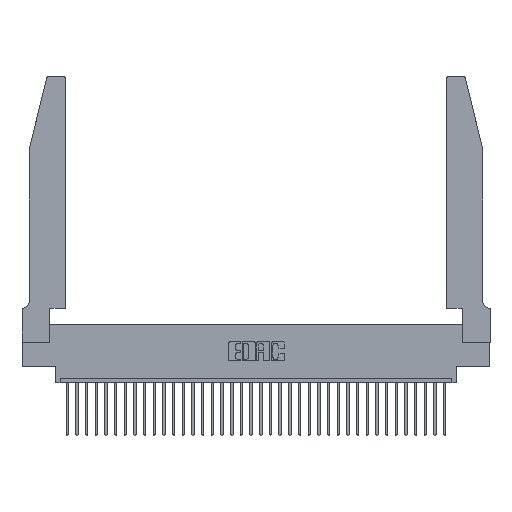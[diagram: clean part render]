
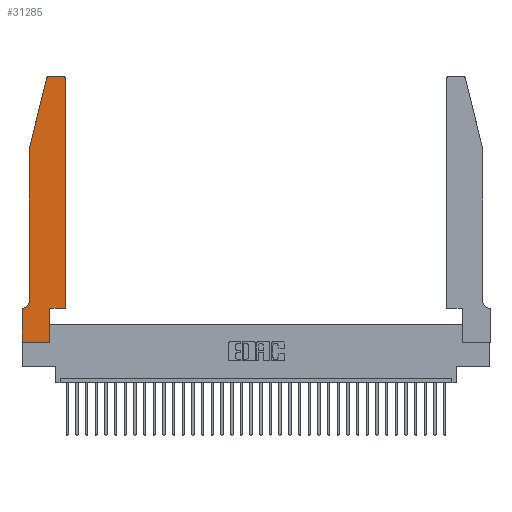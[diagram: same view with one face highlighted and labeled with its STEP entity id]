
A CAD part, top view. The second image highlights one B-rep face of the part: STEP entity #31285.
In plain terms, the highlighted planar face has unit normal (0, 0, 1).
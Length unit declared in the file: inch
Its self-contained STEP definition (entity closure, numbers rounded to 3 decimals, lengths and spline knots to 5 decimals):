
#477 = VECTOR ( 'NONE', #29769, 39.37008 ) ;
#1141 = ORIENTED_EDGE ( 'NONE', *, *, #14739, .T. ) ;
#1378 = EDGE_CURVE ( 'NONE', #14577, #11695, #32129, .T. ) ;
#1543 = EDGE_CURVE ( 'NONE', #13405, #30024, #4927, .T. ) ;
#3015 = DIRECTION ( 'NONE',  ( 0., -1., 0. ) ) ;
#3375 = ORIENTED_EDGE ( 'NONE', *, *, #1543, .T. ) ;
#3447 = CARTESIAN_POINT ( 'NONE',  ( 0.0755, 2., 0.37 ) ) ;
#3746 = EDGE_CURVE ( 'NONE', #33230, #19963, #22677, .T. ) ;
#3959 = EDGE_CURVE ( 'NONE', #5600, #13405, #12819, .T. ) ;
#4927 = LINE ( 'NONE', #29411, #30412 ) ;
#5176 = CARTESIAN_POINT ( 'NONE',  ( 0.2605, 2.75, 0.37 ) ) ;
#5201 = CARTESIAN_POINT ( 'NONE',  ( 0.4205, 2.72, 0.37 ) ) ;
#5505 = CARTESIAN_POINT ( 'NONE',  ( 0.4505, 0.35, 0.37 ) ) ;
#5600 = VERTEX_POINT ( 'NONE', #30991 ) ;
#5765 = FACE_OUTER_BOUND ( 'NONE', #14276, .T. ) ;
#5820 = CARTESIAN_POINT ( 'NONE',  ( 0.25487, 2.72718, 0.37 ) ) ;
#6359 = CARTESIAN_POINT ( 'NONE',  ( 0., 0., 0.37 ) ) ;
#6384 = DIRECTION ( 'NONE',  ( 0., 0., 1. ) ) ;
#6611 = VECTOR ( 'NONE', #15570, 39.37008 ) ;
#6626 = DIRECTION ( 'NONE',  ( 1., 0., 0. ) ) ;
#7242 = ORIENTED_EDGE ( 'NONE', *, *, #23865, .T. ) ;
#7427 = CARTESIAN_POINT ( 'NONE',  ( 0., 0., 0.37 ) ) ;
#8271 = CARTESIAN_POINT ( 'NONE',  ( 0.0755, 0.42, 0.37 ) ) ;
#8273 = LINE ( 'NONE', #5176, #6611 ) ;
#8290 = CARTESIAN_POINT ( 'NONE',  ( 0.0055, 0.35, 0.37 ) ) ;
#8699 = EDGE_CURVE ( 'NONE', #32568, #24597, #12041, .T. ) ;
#9006 = EDGE_CURVE ( 'NONE', #24597, #27833, #17996, .T. ) ;
#9577 = DIRECTION ( 'NONE',  ( 0., -1., 0. ) ) ;
#9740 = AXIS2_PLACEMENT_3D ( 'NONE', #5201, #16184, #10768 ) ;
#10243 = EDGE_CURVE ( 'NONE', #19963, #14577, #11085, .T. ) ;
#10768 = DIRECTION ( 'NONE',  ( 1., 0., 0. ) ) ;
#11085 = LINE ( 'NONE', #28602, #31528 ) ;
#11299 = AXIS2_PLACEMENT_3D ( 'NONE', #27992, #6384, #6626 ) ;
#11360 = CARTESIAN_POINT ( 'NONE',  ( 0., 0.35, 0.37 ) ) ;
#11546 = ORIENTED_EDGE ( 'NONE', *, *, #1378, .T. ) ;
#11695 = VERTEX_POINT ( 'NONE', #32673 ) ;
#12041 = CIRCLE ( 'NONE', #25523, 0.03 ) ;
#12495 = VECTOR ( 'NONE', #30322, 39.37008 ) ;
#12645 = CARTESIAN_POINT ( 'NONE',  ( 0.4205, 2.75, 0.37 ) ) ;
#12819 = LINE ( 'NONE', #29457, #25585 ) ;
#13137 = DIRECTION ( 'NONE',  ( 0., 1., 0. ) ) ;
#13267 = VECTOR ( 'NONE', #3015, 39.37008 ) ;
#13405 = VERTEX_POINT ( 'NONE', #5505 ) ;
#13444 = ORIENTED_EDGE ( 'NONE', *, *, #31544, .T. ) ;
#13888 = DIRECTION ( 'NONE',  ( -1., 0., 0. ) ) ;
#13973 = CARTESIAN_POINT ( 'NONE',  ( 0.0755, 2., 0.37 ) ) ;
#14276 = EDGE_LOOP ( 'NONE', ( #13444, #24852, #16416, #14980, #7242, #32585, #15977, #11546, #1141, #22039, #3375, #20726 ) ) ;
#14486 = PLANE ( 'NONE',  #11299 ) ;
#14577 = VERTEX_POINT ( 'NONE', #6359 ) ;
#14739 = EDGE_CURVE ( 'NONE', #11695, #5600, #23574, .T. ) ;
#14888 = DIRECTION ( 'NONE',  ( 1., 0., 0. ) ) ;
#14980 = ORIENTED_EDGE ( 'NONE', *, *, #21917, .T. ) ;
#15570 = DIRECTION ( 'NONE',  ( -1., 0., 0. ) ) ;
#15977 = ORIENTED_EDGE ( 'NONE', *, *, #10243, .T. ) ;
#16184 = DIRECTION ( 'NONE',  ( 0., 0., 1. ) ) ;
#16416 = ORIENTED_EDGE ( 'NONE', *, *, #9006, .T. ) ;
#17996 = LINE ( 'NONE', #27614, #20109 ) ;
#18873 = CARTESIAN_POINT ( 'NONE',  ( 0.0755, 0.35, 0.37 ) ) ;
#19963 = VERTEX_POINT ( 'NONE', #11360 ) ;
#20109 = VECTOR ( 'NONE', #27955, 39.37008 ) ;
#20498 = LINE ( 'NONE', #13973, #13267 ) ;
#20726 = ORIENTED_EDGE ( 'NONE', *, *, #21867, .T. ) ;
#20971 = CARTESIAN_POINT ( 'NONE',  ( 0.4505, 2.72, 0.37 ) ) ;
#21642 = CARTESIAN_POINT ( 'NONE',  ( 0.0055, 0.42, 0.37 ) ) ;
#21867 = EDGE_CURVE ( 'NONE', #30024, #31336, #22625, .T. ) ;
#21917 = EDGE_CURVE ( 'NONE', #27833, #24715, #20498, .T. ) ;
#22039 = ORIENTED_EDGE ( 'NONE', *, *, #3959, .T. ) ;
#22625 = CIRCLE ( 'NONE', #9740, 0.03 ) ;
#22677 = LINE ( 'NONE', #18873, #477 ) ;
#23574 = LINE ( 'NONE', #25326, #12495 ) ;
#23865 = EDGE_CURVE ( 'NONE', #24715, #33230, #35293, .T. ) ;
#24597 = VERTEX_POINT ( 'NONE', #5820 ) ;
#24715 = VERTEX_POINT ( 'NONE', #8271 ) ;
#24852 = ORIENTED_EDGE ( 'NONE', *, *, #8699, .T. ) ;
#25326 = CARTESIAN_POINT ( 'NONE',  ( 0.2865, 0.35, 0.37 ) ) ;
#25523 = AXIS2_PLACEMENT_3D ( 'NONE', #28037, #31150, #14888 ) ;
#25585 = VECTOR ( 'NONE', #32443, 39.37008 ) ;
#27614 = CARTESIAN_POINT ( 'NONE',  ( 0.0755, 2., 0.37 ) ) ;
#27731 = AXIS2_PLACEMENT_3D ( 'NONE', #21642, #33014, #13888 ) ;
#27833 = VERTEX_POINT ( 'NONE', #3447 ) ;
#27955 = DIRECTION ( 'NONE',  ( -0.239, -0.971, 0. ) ) ;
#27992 = CARTESIAN_POINT ( 'NONE',  ( 0., 0.35, 0.37 ) ) ;
#28037 = CARTESIAN_POINT ( 'NONE',  ( 0.284, 2.72, 0.37 ) ) ;
#28300 = VECTOR ( 'NONE', #33597, 39.37008 ) ;
#28602 = CARTESIAN_POINT ( 'NONE',  ( 0., 0., 0.37 ) ) ;
#29411 = CARTESIAN_POINT ( 'NONE',  ( 0.4505, 0.35, 0.37 ) ) ;
#29457 = CARTESIAN_POINT ( 'NONE',  ( 0.4505, 0.35, 0.37 ) ) ;
#29769 = DIRECTION ( 'NONE',  ( -1., 0., 0. ) ) ;
#30024 = VERTEX_POINT ( 'NONE', #20971 ) ;
#30322 = DIRECTION ( 'NONE',  ( 0., 1., 0. ) ) ;
#30412 = VECTOR ( 'NONE', #13137, 39.37008 ) ;
#30991 = CARTESIAN_POINT ( 'NONE',  ( 0.2865, 0.35, 0.37 ) ) ;
#31150 = DIRECTION ( 'NONE',  ( 0., 0., 1. ) ) ;
#31285 = ADVANCED_FACE ( 'NONE', ( #5765 ), #14486, .T. ) ;
#31336 = VERTEX_POINT ( 'NONE', #12645 ) ;
#31528 = VECTOR ( 'NONE', #9577, 39.37008 ) ;
#31544 = EDGE_CURVE ( 'NONE', #31336, #32568, #8273, .T. ) ;
#32129 = LINE ( 'NONE', #7427, #28300 ) ;
#32443 = DIRECTION ( 'NONE',  ( 1., 0., 0. ) ) ;
#32568 = VERTEX_POINT ( 'NONE', #32964 ) ;
#32585 = ORIENTED_EDGE ( 'NONE', *, *, #3746, .T. ) ;
#32673 = CARTESIAN_POINT ( 'NONE',  ( 0.2865, 0., 0.37 ) ) ;
#32964 = CARTESIAN_POINT ( 'NONE',  ( 0.284, 2.75, 0.37 ) ) ;
#33014 = DIRECTION ( 'NONE',  ( 0., 0., -1. ) ) ;
#33230 = VERTEX_POINT ( 'NONE', #8290 ) ;
#33597 = DIRECTION ( 'NONE',  ( 1., 0., 0. ) ) ;
#35293 = CIRCLE ( 'NONE', #27731, 0.07 ) ;
